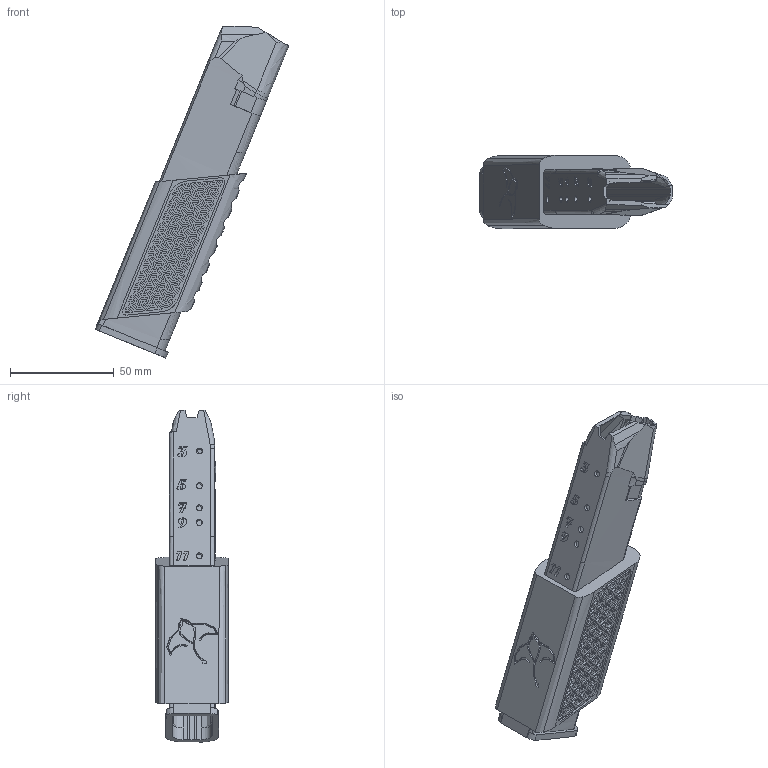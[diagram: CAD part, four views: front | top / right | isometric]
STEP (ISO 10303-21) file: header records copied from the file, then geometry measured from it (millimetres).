
FILE_DESCRIPTION(/* description */ (''),/* implementation_level */ '2;1');
FILE_NAME(/* name */ 'Magazine body.step',/* time_stamp */ '2022-05-12T10:53:44-06:00',/* author */ (''),/* organization */ (''),/* preprocessor_version */ 'ST-DEVELOPER v18.1',/* originating_system */ 'Autodesk Translation Framework v10.10.0.1391',/* authorisation */ '');
FILE_SCHEMA (('AUTOMOTIVE_DESIGN { 1 0 10303 214 3 1 1 }'));
Length unit declared in the file: millimetre
Products named in the file (1): Magazine body
Bounding box: 93.36 x 35.13 x 160.04 mm (x, y, z)
Volume: 70306.6 mm3; surface area: 40678.4 mm2
Topology: 1 solids, 9 shells, 2261 faces, 6099 edges, 4054 vertices
Faces by surface type: plane 2044, bspline 135, cylinder 80, cone 2
Full cylindrical faces by diameter (mm): 3 x5
Entity records: 96380 total; most frequent: CARTESIAN_POINT 43551, ORIENTED_EDGE 12198, DIRECTION 8587, EDGE_CURVE 6099, VERTEX_POINT 4054, LINE 4003, VECTOR 4003, EDGE_LOOP 2475
